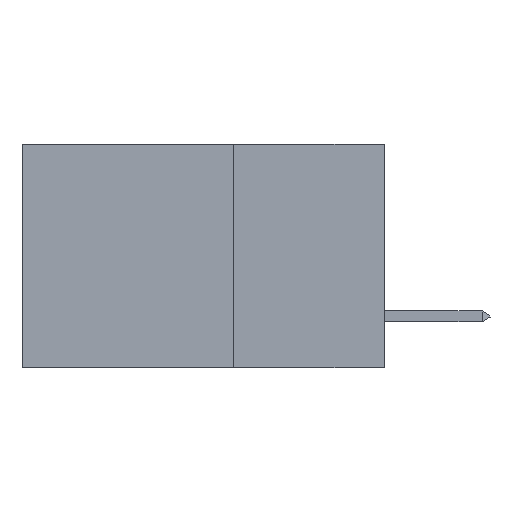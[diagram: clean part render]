
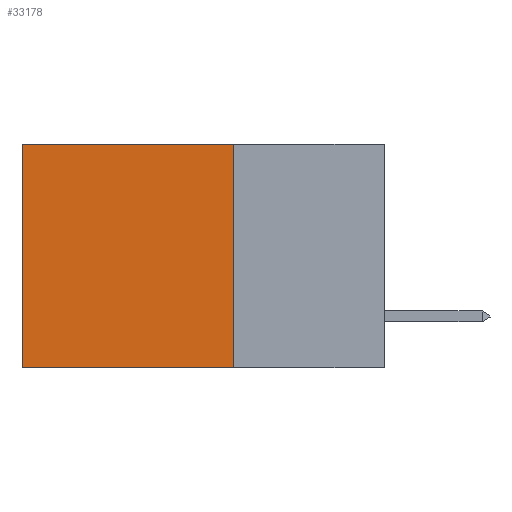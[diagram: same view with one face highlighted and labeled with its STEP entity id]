
A CAD part, left-side view. The second image highlights one B-rep face of the part: STEP entity #33178.
In plain terms, the highlighted planar face has unit normal (-1, 0, 0).
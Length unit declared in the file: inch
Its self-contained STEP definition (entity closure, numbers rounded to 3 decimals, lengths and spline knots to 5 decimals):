
#937 = VERTEX_POINT ( 'NONE', #7372 ) ;
#1653 = VECTOR ( 'NONE', #31207, 39.37008 ) ;
#4002 = LINE ( 'NONE', #35691, #39135 ) ;
#4877 = LINE ( 'NONE', #9413, #9873 ) ;
#5586 = EDGE_CURVE ( 'NONE', #33077, #937, #4002, .T. ) ;
#6807 = EDGE_LOOP ( 'NONE', ( #17231, #35353, #33050, #8973 ) ) ;
#7372 = CARTESIAN_POINT ( 'NONE',  ( 0.2875, 0.6, -0.37 ) ) ;
#7446 = VERTEX_POINT ( 'NONE', #24134 ) ;
#8391 = AXIS2_PLACEMENT_3D ( 'NONE', #24202, #18154, #30772 ) ;
#8973 = ORIENTED_EDGE ( 'NONE', *, *, #18979, .T. ) ;
#9413 = CARTESIAN_POINT ( 'NONE',  ( 0.2875, 0.25, 0. ) ) ;
#9873 = VECTOR ( 'NONE', #35920, 39.37008 ) ;
#13961 = VECTOR ( 'NONE', #28415, 39.37008 ) ;
#15613 = EDGE_CURVE ( 'NONE', #7446, #937, #30988, .T. ) ;
#17231 = ORIENTED_EDGE ( 'NONE', *, *, #5586, .T. ) ;
#18154 = DIRECTION ( 'NONE',  ( 1., 0., 0. ) ) ;
#18979 = EDGE_CURVE ( 'NONE', #40759, #33077, #40346, .T. ) ;
#23366 = DIRECTION ( 'NONE',  ( 0., 0., -1. ) ) ;
#24134 = CARTESIAN_POINT ( 'NONE',  ( 0.2875, 0.25, -0.37 ) ) ;
#24202 = CARTESIAN_POINT ( 'NONE',  ( 0.2875, 0.25, 0. ) ) ;
#24220 = CARTESIAN_POINT ( 'NONE',  ( 0.2875, 0.25, 0. ) ) ;
#24792 = EDGE_CURVE ( 'NONE', #40759, #7446, #4877, .T. ) ;
#25167 = CARTESIAN_POINT ( 'NONE',  ( 0.2875, 0.25, -0.37 ) ) ;
#27549 = PLANE ( 'NONE',  #8391 ) ;
#28415 = DIRECTION ( 'NONE',  ( 0., 1., 0. ) ) ;
#29804 = CARTESIAN_POINT ( 'NONE',  ( 0.2875, 0.6, 0. ) ) ;
#30772 = DIRECTION ( 'NONE',  ( 0., 0., -1. ) ) ;
#30988 = LINE ( 'NONE', #25167, #13961 ) ;
#31207 = DIRECTION ( 'NONE',  ( 0., 1., 0. ) ) ;
#33050 = ORIENTED_EDGE ( 'NONE', *, *, #24792, .F. ) ;
#33077 = VERTEX_POINT ( 'NONE', #29804 ) ;
#33178 = ADVANCED_FACE ( 'NONE', ( #41246 ), #27549, .F. ) ;
#35353 = ORIENTED_EDGE ( 'NONE', *, *, #15613, .F. ) ;
#35691 = CARTESIAN_POINT ( 'NONE',  ( 0.2875, 0.6, 0. ) ) ;
#35920 = DIRECTION ( 'NONE',  ( 0., 0., -1. ) ) ;
#39135 = VECTOR ( 'NONE', #23366, 39.37008 ) ;
#40346 = LINE ( 'NONE', #41320, #1653 ) ;
#40759 = VERTEX_POINT ( 'NONE', #24220 ) ;
#41246 = FACE_OUTER_BOUND ( 'NONE', #6807, .T. ) ;
#41320 = CARTESIAN_POINT ( 'NONE',  ( 0.2875, 0.25, 0. ) ) ;
